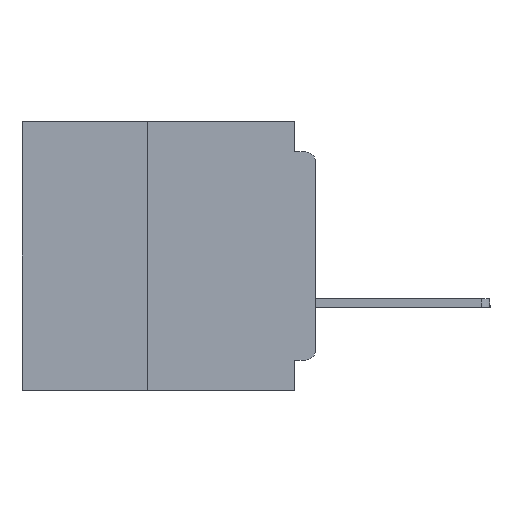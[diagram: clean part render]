
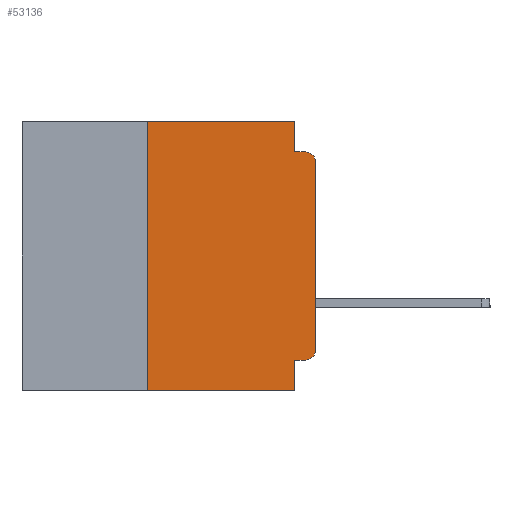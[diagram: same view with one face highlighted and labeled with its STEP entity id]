
A CAD part, left-side view. The second image highlights one B-rep face of the part: STEP entity #53136.
In plain terms, the highlighted planar face has unit normal (-1, 0, 0).
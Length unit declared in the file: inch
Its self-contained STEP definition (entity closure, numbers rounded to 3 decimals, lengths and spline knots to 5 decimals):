
#137 = CARTESIAN_POINT ( 'NONE',  ( 0., 0.031, -0.4 ) ) ;
#1115 = CARTESIAN_POINT ( 'NONE',  ( 0., 0.25, -0.4 ) ) ;
#1669 = LINE ( 'NONE', #39048, #11508 ) ;
#1792 = CARTESIAN_POINT ( 'NONE',  ( 0., 0.015, -0.34 ) ) ;
#3579 = FACE_OUTER_BOUND ( 'NONE', #10386, .T. ) ;
#3628 = LINE ( 'NONE', #15585, #14979 ) ;
#3641 = DIRECTION ( 'NONE',  ( -1., 0., 0. ) ) ;
#3643 = CARTESIAN_POINT ( 'NONE',  ( 0., 0., -0.34 ) ) ;
#4045 = PLANE ( 'NONE',  #58378 ) ;
#4385 = LINE ( 'NONE', #15737, #39856 ) ;
#6672 = DIRECTION ( 'NONE',  ( 0., 0., -1. ) ) ;
#6759 = CIRCLE ( 'NONE', #45624, 0.015 ) ;
#6958 = DIRECTION ( 'NONE',  ( 0., 0., -1. ) ) ;
#7368 = VECTOR ( 'NONE', #52178, 39.37008 ) ;
#8749 = VERTEX_POINT ( 'NONE', #137 ) ;
#8897 = DIRECTION ( 'NONE',  ( 1., 0., 0. ) ) ;
#9168 = VECTOR ( 'NONE', #57129, 39.37008 ) ;
#9341 = VERTEX_POINT ( 'NONE', #24869 ) ;
#10386 = EDGE_LOOP ( 'NONE', ( #10455, #40175, #28205, #18481, #60155, #32075, #13929, #61884, #53544, #21367 ) ) ;
#10455 = ORIENTED_EDGE ( 'NONE', *, *, #43186, .T. ) ;
#10684 = LINE ( 'NONE', #52301, #9168 ) ;
#11002 = CARTESIAN_POINT ( 'NONE',  ( 0., 0.015, -0.045 ) ) ;
#11068 = DIRECTION ( 'NONE',  ( 0., -1., 0. ) ) ;
#11469 = CARTESIAN_POINT ( 'NONE',  ( 0., 0.015, -0.355 ) ) ;
#11508 = VECTOR ( 'NONE', #15028, 39.37008 ) ;
#12167 = CARTESIAN_POINT ( 'NONE',  ( 0., 0.25, 0. ) ) ;
#13929 = ORIENTED_EDGE ( 'NONE', *, *, #14078, .T. ) ;
#14078 = EDGE_CURVE ( 'NONE', #9341, #8749, #10684, .T. ) ;
#14737 = DIRECTION ( 'NONE',  ( 0., 1., 0. ) ) ;
#14979 = VECTOR ( 'NONE', #49230, 39.37008 ) ;
#15028 = DIRECTION ( 'NONE',  ( 0., -1., 0. ) ) ;
#15585 = CARTESIAN_POINT ( 'NONE',  ( 0., 0., 0. ) ) ;
#15737 = CARTESIAN_POINT ( 'NONE',  ( 0., 0., -0.045 ) ) ;
#15740 = DIRECTION ( 'NONE',  ( 0., 0., 1. ) ) ;
#15858 = CARTESIAN_POINT ( 'NONE',  ( 0., 0.031, -0.355 ) ) ;
#18392 = CARTESIAN_POINT ( 'NONE',  ( 0., 0.031, 0. ) ) ;
#18481 = ORIENTED_EDGE ( 'NONE', *, *, #55209, .F. ) ;
#19596 = CARTESIAN_POINT ( 'NONE',  ( 0., 0., -0.355 ) ) ;
#20250 = LINE ( 'NONE', #18392, #7368 ) ;
#20377 = VERTEX_POINT ( 'NONE', #21227 ) ;
#20821 = EDGE_CURVE ( 'NONE', #36966, #35148, #1669, .T. ) ;
#21227 = CARTESIAN_POINT ( 'NONE',  ( 0., 0.031, -0.045 ) ) ;
#21367 = ORIENTED_EDGE ( 'NONE', *, *, #22816, .T. ) ;
#21966 = VECTOR ( 'NONE', #6958, 39.37008 ) ;
#22816 = EDGE_CURVE ( 'NONE', #33400, #35156, #37065, .T. ) ;
#24869 = CARTESIAN_POINT ( 'NONE',  ( 0., 0.25, -0.4 ) ) ;
#25999 = CARTESIAN_POINT ( 'NONE',  ( 0., 0.031, -0.4 ) ) ;
#27766 = CARTESIAN_POINT ( 'NONE',  ( 0., 0.031, 0. ) ) ;
#28205 = ORIENTED_EDGE ( 'NONE', *, *, #54183, .F. ) ;
#31397 = VECTOR ( 'NONE', #15740, 39.37008 ) ;
#32075 = ORIENTED_EDGE ( 'NONE', *, *, #48199, .F. ) ;
#32595 = CARTESIAN_POINT ( 'NONE',  ( 0., 0.015, -0.06 ) ) ;
#33400 = VERTEX_POINT ( 'NONE', #11469 ) ;
#33945 = VERTEX_POINT ( 'NONE', #15858 ) ;
#35148 = VERTEX_POINT ( 'NONE', #27766 ) ;
#35156 = VERTEX_POINT ( 'NONE', #3643 ) ;
#35603 = DIRECTION ( 'NONE',  ( -1., 0., 0. ) ) ;
#36966 = VERTEX_POINT ( 'NONE', #12167 ) ;
#37065 = CIRCLE ( 'NONE', #58693, 0.015 ) ;
#37446 = DIRECTION ( 'NONE',  ( 0., 0., -1. ) ) ;
#38080 = LINE ( 'NONE', #19596, #47838 ) ;
#38098 = EDGE_CURVE ( 'NONE', #33945, #8749, #61696, .T. ) ;
#38173 = VERTEX_POINT ( 'NONE', #41115 ) ;
#39048 = CARTESIAN_POINT ( 'NONE',  ( 0., 0.437, 0. ) ) ;
#39856 = VECTOR ( 'NONE', #11068, 39.37008 ) ;
#40175 = ORIENTED_EDGE ( 'NONE', *, *, #62157, .T. ) ;
#41115 = CARTESIAN_POINT ( 'NONE',  ( 0., 0., -0.06 ) ) ;
#41424 = VERTEX_POINT ( 'NONE', #11002 ) ;
#42628 = DIRECTION ( 'NONE',  ( 0., 0., -1. ) ) ;
#43186 = EDGE_CURVE ( 'NONE', #35156, #38173, #3628, .T. ) ;
#44144 = LINE ( 'NONE', #1115, #31397 ) ;
#45624 = AXIS2_PLACEMENT_3D ( 'NONE', #32595, #3641, #37446 ) ;
#47067 = CARTESIAN_POINT ( 'NONE',  ( 0., 0.437, 0. ) ) ;
#47838 = VECTOR ( 'NONE', #14737, 39.37008 ) ;
#48199 = EDGE_CURVE ( 'NONE', #9341, #36966, #44144, .T. ) ;
#49230 = DIRECTION ( 'NONE',  ( 0., 0., 1. ) ) ;
#52178 = DIRECTION ( 'NONE',  ( 0., 0., -1. ) ) ;
#52301 = CARTESIAN_POINT ( 'NONE',  ( 0., 0.437, -0.4 ) ) ;
#53136 = ADVANCED_FACE ( 'NONE', ( #3579 ), #4045, .F. ) ;
#53544 = ORIENTED_EDGE ( 'NONE', *, *, #57021, .F. ) ;
#54183 = EDGE_CURVE ( 'NONE', #20377, #41424, #4385, .T. ) ;
#55209 = EDGE_CURVE ( 'NONE', #35148, #20377, #20250, .T. ) ;
#57021 = EDGE_CURVE ( 'NONE', #33400, #33945, #38080, .T. ) ;
#57129 = DIRECTION ( 'NONE',  ( 0., -1., 0. ) ) ;
#58378 = AXIS2_PLACEMENT_3D ( 'NONE', #47067, #8897, #42628 ) ;
#58693 = AXIS2_PLACEMENT_3D ( 'NONE', #1792, #35603, #6672 ) ;
#60155 = ORIENTED_EDGE ( 'NONE', *, *, #20821, .F. ) ;
#61696 = LINE ( 'NONE', #25999, #21966 ) ;
#61884 = ORIENTED_EDGE ( 'NONE', *, *, #38098, .F. ) ;
#62157 = EDGE_CURVE ( 'NONE', #38173, #41424, #6759, .T. ) ;
